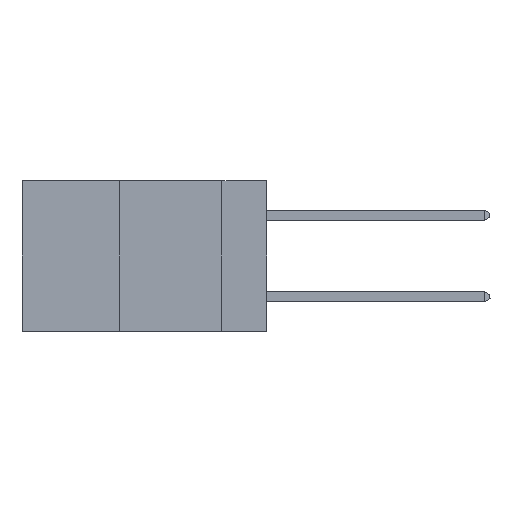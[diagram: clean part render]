
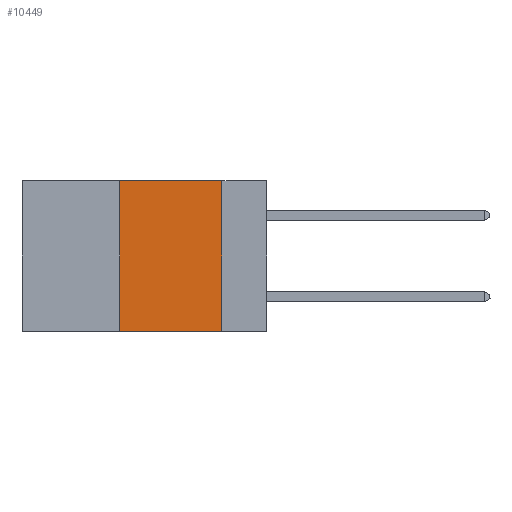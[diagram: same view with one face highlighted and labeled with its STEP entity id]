
A CAD part, left-side view. The second image highlights one B-rep face of the part: STEP entity #10449.
In plain terms, the highlighted planar face has unit normal (-1, 0, 0).
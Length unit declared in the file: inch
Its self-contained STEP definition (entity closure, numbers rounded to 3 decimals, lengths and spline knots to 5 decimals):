
#8 = DIRECTION ( 'NONE',  ( 0., -1., 0. ) ) ;
#632 = DIRECTION ( 'NONE',  ( 0., 0., -1. ) ) ;
#691 = EDGE_CURVE ( 'NONE', #8183, #5385, #4876, .T. ) ;
#695 = CARTESIAN_POINT ( 'NONE',  ( 0., 0.11, 0. ) ) ;
#1654 = ORIENTED_EDGE ( 'NONE', *, *, #2585, .T. ) ;
#1738 = CARTESIAN_POINT ( 'NONE',  ( 0., 0.36, 0. ) ) ;
#2585 = EDGE_CURVE ( 'NONE', #6194, #5385, #6945, .T. ) ;
#3280 = EDGE_CURVE ( 'NONE', #14614, #8183, #16934, .T. ) ;
#3518 = EDGE_CURVE ( 'NONE', #6194, #14614, #16717, .T. ) ;
#3568 = PLANE ( 'NONE',  #7487 ) ;
#4876 = LINE ( 'NONE', #695, #12081 ) ;
#5385 = VERTEX_POINT ( 'NONE', #15147 ) ;
#6194 = VERTEX_POINT ( 'NONE', #14754 ) ;
#6332 = DIRECTION ( 'NONE',  ( 0., 0., -1. ) ) ;
#6466 = FACE_OUTER_BOUND ( 'NONE', #7034, .T. ) ;
#6568 = CARTESIAN_POINT ( 'NONE',  ( 0., 0.6, -0.37 ) ) ;
#6945 = LINE ( 'NONE', #6568, #10117 ) ;
#7034 = EDGE_LOOP ( 'NONE', ( #13422, #16244, #14611, #1654 ) ) ;
#7487 = AXIS2_PLACEMENT_3D ( 'NONE', #8998, #14395, #6332 ) ;
#8183 = VERTEX_POINT ( 'NONE', #12433 ) ;
#8998 = CARTESIAN_POINT ( 'NONE',  ( 0., 0.6, 0. ) ) ;
#9664 = VECTOR ( 'NONE', #12091, 39.37008 ) ;
#10006 = CARTESIAN_POINT ( 'NONE',  ( 0., 0.6, 0. ) ) ;
#10117 = VECTOR ( 'NONE', #8, 39.37008 ) ;
#10295 = VECTOR ( 'NONE', #13234, 39.37008 ) ;
#10449 = ADVANCED_FACE ( 'NONE', ( #6466 ), #3568, .F. ) ;
#12035 = CARTESIAN_POINT ( 'NONE',  ( 0., 0.36, 0. ) ) ;
#12081 = VECTOR ( 'NONE', #632, 39.37008 ) ;
#12091 = DIRECTION ( 'NONE',  ( 0., 0., 1. ) ) ;
#12433 = CARTESIAN_POINT ( 'NONE',  ( 0., 0.11, 0. ) ) ;
#13234 = DIRECTION ( 'NONE',  ( 0., -1., 0. ) ) ;
#13422 = ORIENTED_EDGE ( 'NONE', *, *, #691, .F. ) ;
#14395 = DIRECTION ( 'NONE',  ( 1., 0., 0. ) ) ;
#14611 = ORIENTED_EDGE ( 'NONE', *, *, #3518, .F. ) ;
#14614 = VERTEX_POINT ( 'NONE', #1738 ) ;
#14754 = CARTESIAN_POINT ( 'NONE',  ( 0., 0.36, -0.37 ) ) ;
#15147 = CARTESIAN_POINT ( 'NONE',  ( 0., 0.11, -0.37 ) ) ;
#16244 = ORIENTED_EDGE ( 'NONE', *, *, #3280, .F. ) ;
#16717 = LINE ( 'NONE', #12035, #9664 ) ;
#16934 = LINE ( 'NONE', #10006, #10295 ) ;
